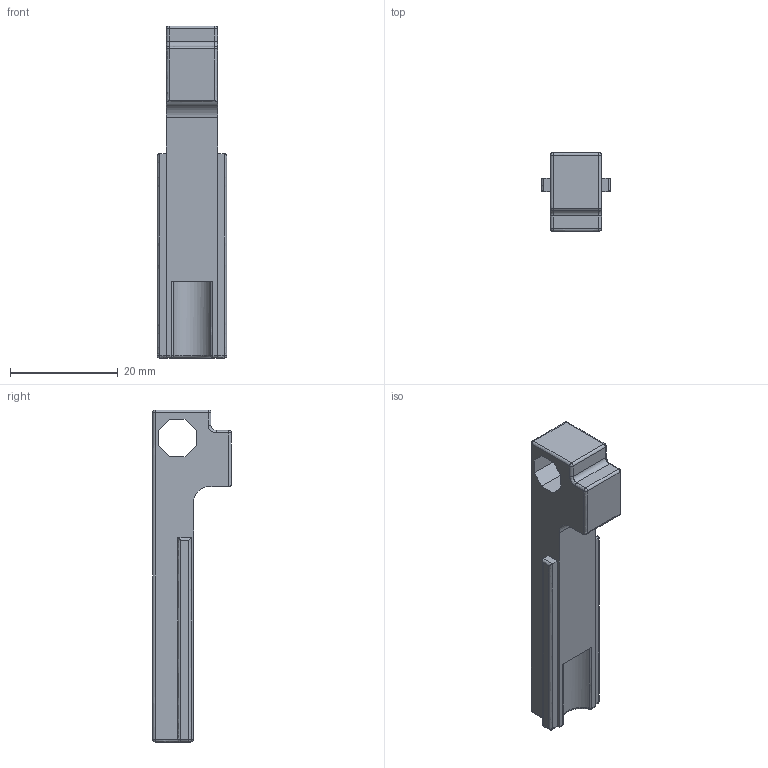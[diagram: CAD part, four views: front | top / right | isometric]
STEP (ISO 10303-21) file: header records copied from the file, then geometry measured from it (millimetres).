
FILE_DESCRIPTION (( 'STEP AP214' ), '1' );
FILE_NAME ('Charging Block.step', '2019-12-18T03:07:19', ( '' ), ( '' ), 'SwSTEP 2.0', 'SolidWorks 2019', '' );
FILE_SCHEMA (( 'AUTOMOTIVE_DESIGN' ));
Length unit declared in the file: millimetre
Products named in the file (1): Charging Block
Bounding box: 12.98 x 14.63 x 61.75 mm (x, y, z)
Volume: 5025.2 mm3; surface area: 2912.7 mm2
Topology: 1 solids, 1 shells, 82 faces, 196 edges, 102 vertices
Faces by surface type: bspline 38, plane 27, sphere 14, cylinder 3
Entity records: 3189 total; most frequent: CARTESIAN_POINT 1813, ORIENTED_EDGE 364, EDGE_CURVE 182, DIRECTION 143, B_SPLINE_CURVE_WITH_KNOTS 112, VERTEX_POINT 102, EDGE_LOOP 84, ADVANCED_FACE 82
